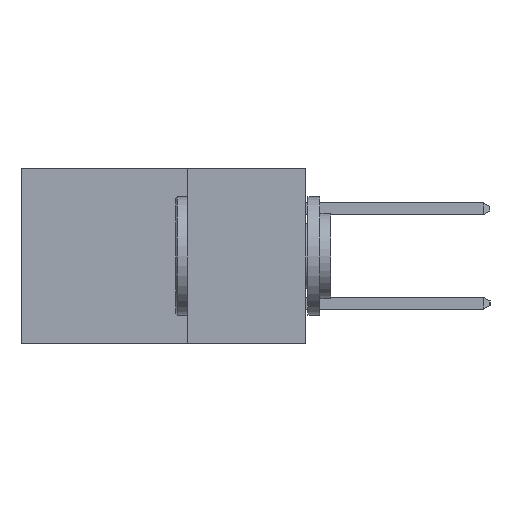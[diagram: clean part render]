
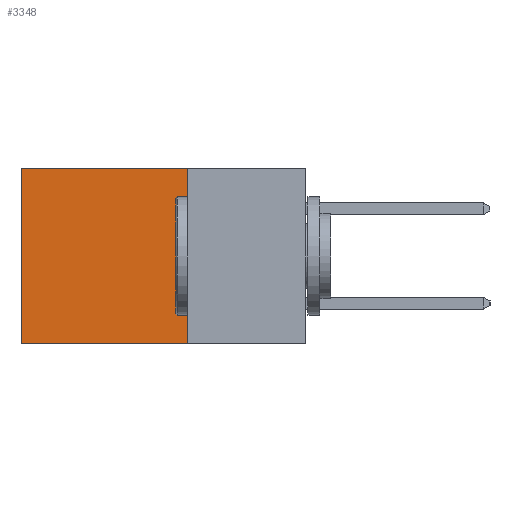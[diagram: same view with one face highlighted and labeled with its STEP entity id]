
A CAD part, left-side view. The second image highlights one B-rep face of the part: STEP entity #3348.
In plain terms, the highlighted planar face has unit normal (-1, 0, 0).
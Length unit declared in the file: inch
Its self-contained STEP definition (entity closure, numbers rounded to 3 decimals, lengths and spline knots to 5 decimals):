
#122 = VECTOR ( 'NONE', #13126, 39.37008 ) ;
#562 = LINE ( 'NONE', #14454, #8305 ) ;
#1861 = VERTEX_POINT ( 'NONE', #8114 ) ;
#2726 = CARTESIAN_POINT ( 'NONE',  ( 0.2615, 0.6, -0.37 ) ) ;
#3348 = ADVANCED_FACE ( 'NONE', ( #9019 ), #7587, .F. ) ;
#5062 = VERTEX_POINT ( 'NONE', #7243 ) ;
#5116 = VECTOR ( 'NONE', #6465, 39.37008 ) ;
#6465 = DIRECTION ( 'NONE',  ( 0., 1., 0. ) ) ;
#7243 = CARTESIAN_POINT ( 'NONE',  ( 0.2615, 0.25, -0.37 ) ) ;
#7587 = PLANE ( 'NONE',  #18921 ) ;
#7607 = CARTESIAN_POINT ( 'NONE',  ( 0.2615, 0.25, -0.37 ) ) ;
#8114 = CARTESIAN_POINT ( 'NONE',  ( 0.2615, 0.25, 0. ) ) ;
#8305 = VECTOR ( 'NONE', #16005, 39.37008 ) ;
#9019 = FACE_OUTER_BOUND ( 'NONE', #15856, .T. ) ;
#9234 = EDGE_CURVE ( 'NONE', #1861, #5062, #562, .T. ) ;
#9354 = VERTEX_POINT ( 'NONE', #2726 ) ;
#10116 = VECTOR ( 'NONE', #12321, 39.37008 ) ;
#10134 = EDGE_CURVE ( 'NONE', #13386, #9354, #17967, .T. ) ;
#11646 = CARTESIAN_POINT ( 'NONE',  ( 0.2615, 0.25, 0. ) ) ;
#12045 = ORIENTED_EDGE ( 'NONE', *, *, #18081, .F. ) ;
#12064 = DIRECTION ( 'NONE',  ( 0., 0., -1. ) ) ;
#12130 = DIRECTION ( 'NONE',  ( 1., 0., 0. ) ) ;
#12319 = LINE ( 'NONE', #11646, #122 ) ;
#12321 = DIRECTION ( 'NONE',  ( 0., 0., -1. ) ) ;
#13126 = DIRECTION ( 'NONE',  ( 0., 1., 0. ) ) ;
#13386 = VERTEX_POINT ( 'NONE', #13848 ) ;
#13738 = EDGE_CURVE ( 'NONE', #1861, #13386, #12319, .T. ) ;
#13848 = CARTESIAN_POINT ( 'NONE',  ( 0.2615, 0.6, 0. ) ) ;
#13909 = CARTESIAN_POINT ( 'NONE',  ( 0.2615, 0.25, -0.37 ) ) ;
#14454 = CARTESIAN_POINT ( 'NONE',  ( 0.2615, 0.25, -0.37 ) ) ;
#15340 = ORIENTED_EDGE ( 'NONE', *, *, #10134, .T. ) ;
#15856 = EDGE_LOOP ( 'NONE', ( #15340, #12045, #16968, #19084 ) ) ;
#16005 = DIRECTION ( 'NONE',  ( 0., 0., -1. ) ) ;
#16633 = LINE ( 'NONE', #13909, #5116 ) ;
#16968 = ORIENTED_EDGE ( 'NONE', *, *, #9234, .F. ) ;
#17967 = LINE ( 'NONE', #18179, #10116 ) ;
#18081 = EDGE_CURVE ( 'NONE', #5062, #9354, #16633, .T. ) ;
#18179 = CARTESIAN_POINT ( 'NONE',  ( 0.2615, 0.6, -0.37 ) ) ;
#18921 = AXIS2_PLACEMENT_3D ( 'NONE', #7607, #12130, #12064 ) ;
#19084 = ORIENTED_EDGE ( 'NONE', *, *, #13738, .T. ) ;
